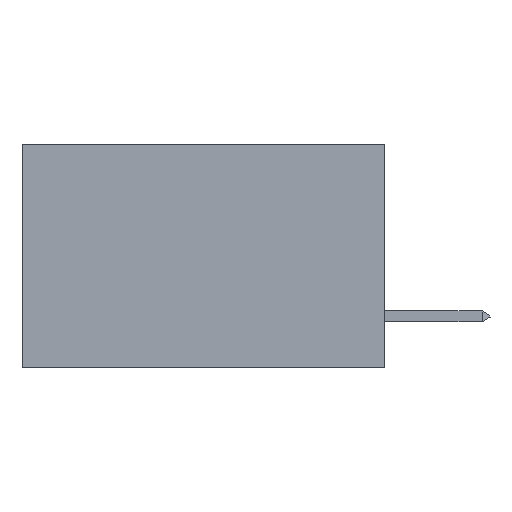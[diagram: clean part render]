
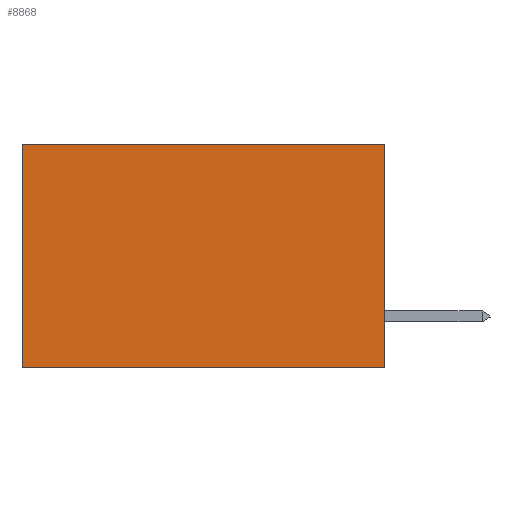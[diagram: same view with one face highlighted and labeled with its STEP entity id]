
A CAD part, left-side view. The second image highlights one B-rep face of the part: STEP entity #8868.
In plain terms, the highlighted planar face has unit normal (-1, 0, 0).
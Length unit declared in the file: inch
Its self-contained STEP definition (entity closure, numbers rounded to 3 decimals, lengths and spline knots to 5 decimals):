
#445 = VERTEX_POINT ( 'NONE', #2938 ) ;
#1125 = DIRECTION ( 'NONE',  ( 0., 0., -1. ) ) ;
#1305 = AXIS2_PLACEMENT_3D ( 'NONE', #6730, #10647, #1125 ) ;
#1566 = VERTEX_POINT ( 'NONE', #5418 ) ;
#1659 = DIRECTION ( 'NONE',  ( 0., 1., 0. ) ) ;
#1756 = FACE_OUTER_BOUND ( 'NONE', #3057, .T. ) ;
#1945 = CARTESIAN_POINT ( 'NONE',  ( 0.2875, 0., 0. ) ) ;
#2092 = PLANE ( 'NONE',  #1305 ) ;
#2526 = VECTOR ( 'NONE', #11394, 39.37008 ) ;
#2790 = LINE ( 'NONE', #7827, #4995 ) ;
#2938 = CARTESIAN_POINT ( 'NONE',  ( 0.2875, 0.6, -0.37 ) ) ;
#3057 = EDGE_LOOP ( 'NONE', ( #9884, #10372, #7005, #3382 ) ) ;
#3189 = DIRECTION ( 'NONE',  ( 0., 0., -1. ) ) ;
#3265 = VECTOR ( 'NONE', #10862, 39.37008 ) ;
#3382 = ORIENTED_EDGE ( 'NONE', *, *, #7639, .T. ) ;
#4995 = VECTOR ( 'NONE', #3189, 39.37008 ) ;
#5143 = CARTESIAN_POINT ( 'NONE',  ( 0.2875, 0.6, 0. ) ) ;
#5418 = CARTESIAN_POINT ( 'NONE',  ( 0.2875, 0., 0. ) ) ;
#5725 = VERTEX_POINT ( 'NONE', #8919 ) ;
#6730 = CARTESIAN_POINT ( 'NONE',  ( 0.2875, 0., 0. ) ) ;
#6950 = EDGE_CURVE ( 'NONE', #5725, #445, #10678, .T. ) ;
#7005 = ORIENTED_EDGE ( 'NONE', *, *, #9408, .F. ) ;
#7051 = LINE ( 'NONE', #5143, #3265 ) ;
#7639 = EDGE_CURVE ( 'NONE', #1566, #11528, #10808, .T. ) ;
#7827 = CARTESIAN_POINT ( 'NONE',  ( 0.2875, 0., 0. ) ) ;
#8868 = ADVANCED_FACE ( 'NONE', ( #1756 ), #2092, .F. ) ;
#8919 = CARTESIAN_POINT ( 'NONE',  ( 0.2875, 0., -0.37 ) ) ;
#8953 = CARTESIAN_POINT ( 'NONE',  ( 0.2875, 0.6, 0. ) ) ;
#9039 = VECTOR ( 'NONE', #1659, 39.37008 ) ;
#9049 = EDGE_CURVE ( 'NONE', #11528, #445, #7051, .T. ) ;
#9408 = EDGE_CURVE ( 'NONE', #1566, #5725, #2790, .T. ) ;
#9884 = ORIENTED_EDGE ( 'NONE', *, *, #9049, .T. ) ;
#10372 = ORIENTED_EDGE ( 'NONE', *, *, #6950, .F. ) ;
#10647 = DIRECTION ( 'NONE',  ( 1., 0., 0. ) ) ;
#10678 = LINE ( 'NONE', #11905, #9039 ) ;
#10808 = LINE ( 'NONE', #1945, #2526 ) ;
#10862 = DIRECTION ( 'NONE',  ( 0., 0., -1. ) ) ;
#11394 = DIRECTION ( 'NONE',  ( 0., 1., 0. ) ) ;
#11528 = VERTEX_POINT ( 'NONE', #8953 ) ;
#11905 = CARTESIAN_POINT ( 'NONE',  ( 0.2875, 0., -0.37 ) ) ;
